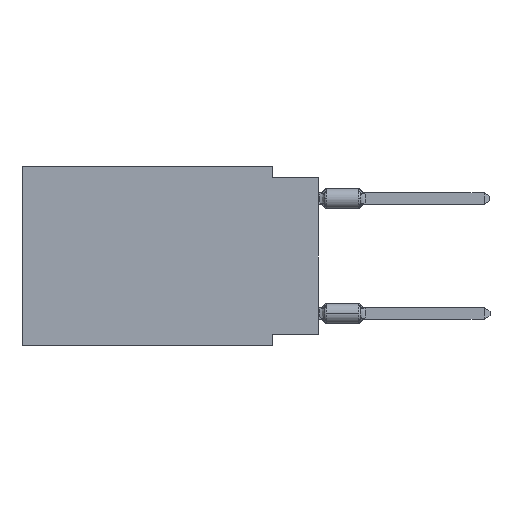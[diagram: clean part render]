
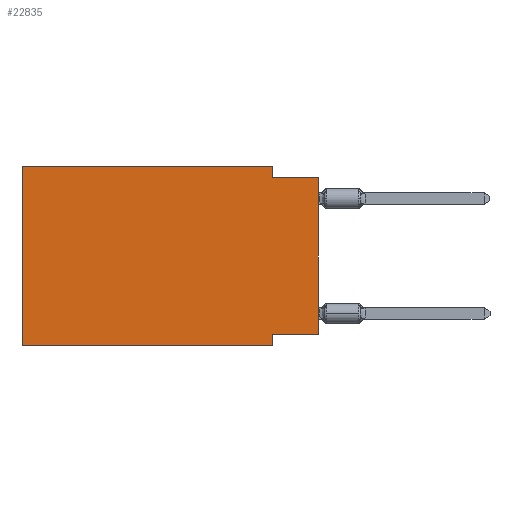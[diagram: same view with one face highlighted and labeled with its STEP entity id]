
A CAD part, left-side view. The second image highlights one B-rep face of the part: STEP entity #22835.
In plain terms, the highlighted planar face has unit normal (-1, 0, 0).
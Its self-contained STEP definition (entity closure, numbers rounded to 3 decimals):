
#11 = EDGE_LOOP ( 'NONE', ( #17978, #9795, #13782, #2735, #787, #19347, #16538, #3579 ) ) ;
#273 = VERTEX_POINT ( 'NONE', #20598 ) ;
#754 = CARTESIAN_POINT ( 'NONE',  ( 0., 16.383, 0. ) ) ;
#787 = ORIENTED_EDGE ( 'NONE', *, *, #2985, .F. ) ;
#815 = LINE ( 'NONE', #8635, #16019 ) ;
#819 = LINE ( 'NONE', #21244, #23483 ) ;
#917 = EDGE_CURVE ( 'NONE', #7764, #273, #3063, .T. ) ;
#988 = CARTESIAN_POINT ( 'NONE',  ( 0., 0., -0.635 ) ) ;
#1443 = EDGE_CURVE ( 'NONE', #15015, #22627, #18413, .T. ) ;
#1669 = CARTESIAN_POINT ( 'NONE',  ( 0., 2.54, 0. ) ) ;
#1855 = VECTOR ( 'NONE', #21466, 1000. ) ;
#1971 = DIRECTION ( 'NONE',  ( 0., 1., 0. ) ) ;
#2467 = FACE_OUTER_BOUND ( 'NONE', #11, .T. ) ;
#2735 = ORIENTED_EDGE ( 'NONE', *, *, #7085, .F. ) ;
#2985 = EDGE_CURVE ( 'NONE', #7764, #12417, #8016, .T. ) ;
#3063 = LINE ( 'NONE', #10521, #19700 ) ;
#3579 = ORIENTED_EDGE ( 'NONE', *, *, #9675, .F. ) ;
#3719 = AXIS2_PLACEMENT_3D ( 'NONE', #754, #19459, #19578 ) ;
#4378 = VERTEX_POINT ( 'NONE', #24032 ) ;
#5074 = EDGE_CURVE ( 'NONE', #13285, #273, #14325, .T. ) ;
#6225 = CARTESIAN_POINT ( 'NONE',  ( 0., 16.383, -9.906 ) ) ;
#6829 = CARTESIAN_POINT ( 'NONE',  ( 0., 0., 0. ) ) ;
#7085 = EDGE_CURVE ( 'NONE', #12417, #15015, #815, .T. ) ;
#7211 = VECTOR ( 'NONE', #23322, 1000. ) ;
#7448 = CARTESIAN_POINT ( 'NONE',  ( 0., 0., -9.271 ) ) ;
#7764 = VERTEX_POINT ( 'NONE', #6225 ) ;
#8016 = LINE ( 'NONE', #15498, #1855 ) ;
#8075 = PLANE ( 'NONE',  #3719 ) ;
#8302 = DIRECTION ( 'NONE',  ( 0., 0., 1. ) ) ;
#8635 = CARTESIAN_POINT ( 'NONE',  ( 0., 16.383, 0. ) ) ;
#9426 = CARTESIAN_POINT ( 'NONE',  ( 0., 16.383, 0. ) ) ;
#9675 = EDGE_CURVE ( 'NONE', #4378, #13285, #18712, .T. ) ;
#9795 = ORIENTED_EDGE ( 'NONE', *, *, #16620, .F. ) ;
#10429 = CARTESIAN_POINT ( 'NONE',  ( 0., 2.54, -0.635 ) ) ;
#10521 = CARTESIAN_POINT ( 'NONE',  ( 0., 16.383, -9.906 ) ) ;
#12417 = VERTEX_POINT ( 'NONE', #9426 ) ;
#12927 = VECTOR ( 'NONE', #1971, 1000. ) ;
#13285 = VERTEX_POINT ( 'NONE', #17876 ) ;
#13621 = EDGE_CURVE ( 'NONE', #4378, #20135, #23465, .T. ) ;
#13782 = ORIENTED_EDGE ( 'NONE', *, *, #1443, .F. ) ;
#14325 = LINE ( 'NONE', #14690, #17810 ) ;
#14690 = CARTESIAN_POINT ( 'NONE',  ( 0., 2.54, -9.906 ) ) ;
#15015 = VERTEX_POINT ( 'NONE', #22599 ) ;
#15498 = CARTESIAN_POINT ( 'NONE',  ( 0., 16.383, 0. ) ) ;
#16019 = VECTOR ( 'NONE', #19523, 1000. ) ;
#16538 = ORIENTED_EDGE ( 'NONE', *, *, #5074, .F. ) ;
#16620 = EDGE_CURVE ( 'NONE', #22627, #20135, #819, .T. ) ;
#17810 = VECTOR ( 'NONE', #20317, 1000. ) ;
#17854 = DIRECTION ( 'NONE',  ( 0., -1., 0. ) ) ;
#17876 = CARTESIAN_POINT ( 'NONE',  ( 0., 2.54, -9.271 ) ) ;
#17978 = ORIENTED_EDGE ( 'NONE', *, *, #13621, .T. ) ;
#18413 = LINE ( 'NONE', #1669, #7211 ) ;
#18712 = LINE ( 'NONE', #7448, #12927 ) ;
#19347 = ORIENTED_EDGE ( 'NONE', *, *, #917, .T. ) ;
#19459 = DIRECTION ( 'NONE',  ( 1., 0., 0. ) ) ;
#19523 = DIRECTION ( 'NONE',  ( 0., -1., 0. ) ) ;
#19531 = DIRECTION ( 'NONE',  ( 0., -1., 0. ) ) ;
#19578 = DIRECTION ( 'NONE',  ( 0., 0., -1. ) ) ;
#19700 = VECTOR ( 'NONE', #17854, 1000. ) ;
#20135 = VERTEX_POINT ( 'NONE', #988 ) ;
#20317 = DIRECTION ( 'NONE',  ( 0., 0., -1. ) ) ;
#20598 = CARTESIAN_POINT ( 'NONE',  ( 0., 2.54, -9.906 ) ) ;
#21244 = CARTESIAN_POINT ( 'NONE',  ( 0., 0., -0.635 ) ) ;
#21466 = DIRECTION ( 'NONE',  ( 0., 0., 1. ) ) ;
#22599 = CARTESIAN_POINT ( 'NONE',  ( 0., 2.54, 0. ) ) ;
#22627 = VERTEX_POINT ( 'NONE', #10429 ) ;
#22835 = ADVANCED_FACE ( 'NONE', ( #2467 ), #8075, .F. ) ;
#23322 = DIRECTION ( 'NONE',  ( 0., 0., -1. ) ) ;
#23465 = LINE ( 'NONE', #6829, #24183 ) ;
#23483 = VECTOR ( 'NONE', #19531, 1000. ) ;
#24032 = CARTESIAN_POINT ( 'NONE',  ( 0., 0., -9.271 ) ) ;
#24183 = VECTOR ( 'NONE', #8302, 1000. ) ;
